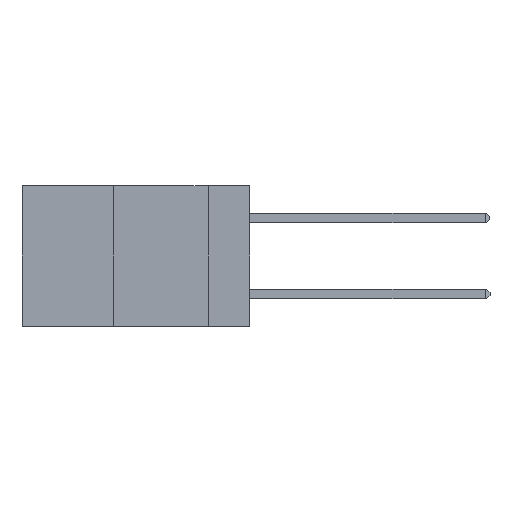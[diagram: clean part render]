
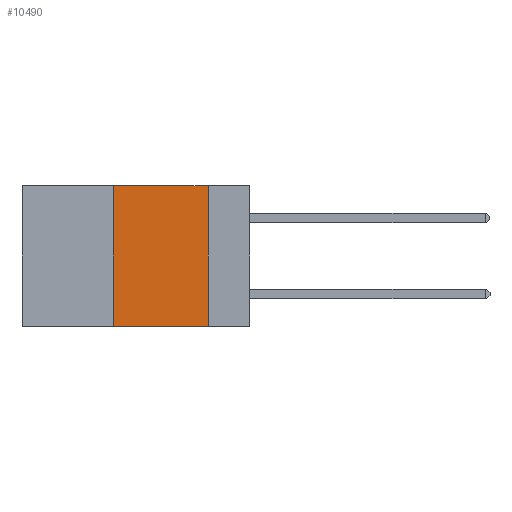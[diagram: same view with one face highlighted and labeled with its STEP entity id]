
A CAD part, left-side view. The second image highlights one B-rep face of the part: STEP entity #10490.
In plain terms, the highlighted planar face has unit normal (-1, 0, 0).
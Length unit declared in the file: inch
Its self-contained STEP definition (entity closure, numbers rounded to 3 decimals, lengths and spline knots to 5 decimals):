
#337 = EDGE_CURVE ( 'NONE', #13992, #12572, #6600, .T. ) ;
#1386 = VECTOR ( 'NONE', #5766, 39.37008 ) ;
#2928 = EDGE_CURVE ( 'NONE', #21226, #13992, #18189, .T. ) ;
#3233 = EDGE_CURVE ( 'NONE', #12039, #12572, #20706, .T. ) ;
#5070 = CARTESIAN_POINT ( 'NONE',  ( 0., 0.36, -0.37 ) ) ;
#5766 = DIRECTION ( 'NONE',  ( 0., 0., -1. ) ) ;
#6600 = LINE ( 'NONE', #19203, #1386 ) ;
#6632 = DIRECTION ( 'NONE',  ( 0., -1., 0. ) ) ;
#7364 = VECTOR ( 'NONE', #20746, 39.37008 ) ;
#7504 = DIRECTION ( 'NONE',  ( 1., 0., 0. ) ) ;
#8023 = CARTESIAN_POINT ( 'NONE',  ( 0., 0.11, -0.37 ) ) ;
#8194 = CARTESIAN_POINT ( 'NONE',  ( 0., 0.36, 0. ) ) ;
#8276 = CARTESIAN_POINT ( 'NONE',  ( 0., 0.6, 0. ) ) ;
#10047 = EDGE_CURVE ( 'NONE', #12039, #21226, #21106, .T. ) ;
#10490 = ADVANCED_FACE ( 'NONE', ( #15668 ), #10752, .F. ) ;
#10702 = CARTESIAN_POINT ( 'NONE',  ( 0., 0.6, -0.37 ) ) ;
#10752 = PLANE ( 'NONE',  #19190 ) ;
#11431 = DIRECTION ( 'NONE',  ( 0., 0., 1. ) ) ;
#11715 = ORIENTED_EDGE ( 'NONE', *, *, #3233, .T. ) ;
#12039 = VERTEX_POINT ( 'NONE', #5070 ) ;
#12572 = VERTEX_POINT ( 'NONE', #8023 ) ;
#13443 = CARTESIAN_POINT ( 'NONE',  ( 0., 0.11, 0. ) ) ;
#13661 = VECTOR ( 'NONE', #6632, 39.37008 ) ;
#13992 = VERTEX_POINT ( 'NONE', #13443 ) ;
#15668 = FACE_OUTER_BOUND ( 'NONE', #20147, .T. ) ;
#15686 = VECTOR ( 'NONE', #11431, 39.37008 ) ;
#17585 = CARTESIAN_POINT ( 'NONE',  ( 0., 0.6, 0. ) ) ;
#17818 = ORIENTED_EDGE ( 'NONE', *, *, #2928, .F. ) ;
#18132 = ORIENTED_EDGE ( 'NONE', *, *, #10047, .F. ) ;
#18189 = LINE ( 'NONE', #8276, #13661 ) ;
#18303 = CARTESIAN_POINT ( 'NONE',  ( 0., 0.36, 0. ) ) ;
#19190 = AXIS2_PLACEMENT_3D ( 'NONE', #17585, #7504, #19234 ) ;
#19203 = CARTESIAN_POINT ( 'NONE',  ( 0., 0.11, 0. ) ) ;
#19212 = ORIENTED_EDGE ( 'NONE', *, *, #337, .F. ) ;
#19234 = DIRECTION ( 'NONE',  ( 0., 0., -1. ) ) ;
#20147 = EDGE_LOOP ( 'NONE', ( #19212, #17818, #18132, #11715 ) ) ;
#20706 = LINE ( 'NONE', #10702, #7364 ) ;
#20746 = DIRECTION ( 'NONE',  ( 0., -1., 0. ) ) ;
#21106 = LINE ( 'NONE', #8194, #15686 ) ;
#21226 = VERTEX_POINT ( 'NONE', #18303 ) ;
